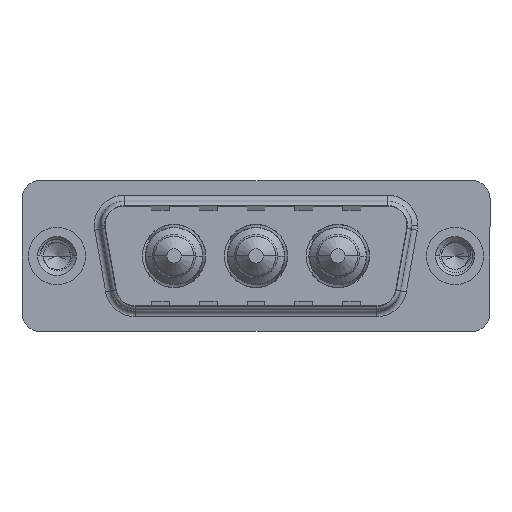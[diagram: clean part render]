
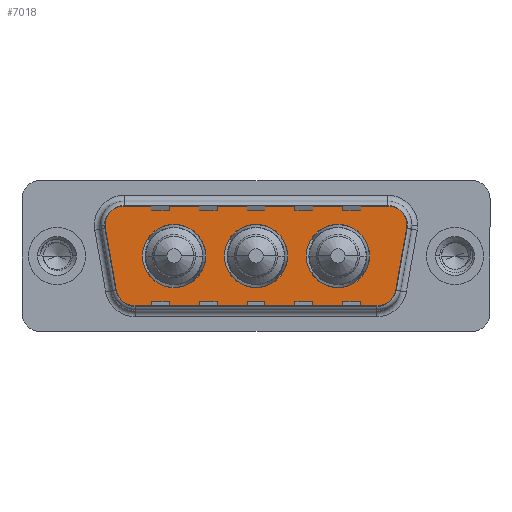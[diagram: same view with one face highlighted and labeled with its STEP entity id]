
A CAD part, top view. The second image highlights one B-rep face of the part: STEP entity #7018.
In plain terms, the highlighted planar face has unit normal (0, 0, 1).
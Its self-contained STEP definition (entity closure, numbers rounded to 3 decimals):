
#6 = ORIENTED_EDGE ( 'NONE', *, *, #17753, .F. ) ;
#255 = CARTESIAN_POINT ( 'NONE',  ( 27.889, 2.9, 0. ) ) ;
#508 = CARTESIAN_POINT ( 'NONE',  ( 26.866, -2.9, 0. ) ) ;
#738 = DIRECTION ( 'NONE',  ( 1., 0., 0. ) ) ;
#1207 = FACE_OUTER_BOUND ( 'NONE', #15820, .T. ) ;
#1309 = DIRECTION ( 'NONE',  ( 0., 0., 1. ) ) ;
#1319 = CARTESIAN_POINT ( 'NONE',  ( 3.441, 2.553, 0. ) ) ;
#1426 = CARTESIAN_POINT ( 'NONE',  ( 28.836, -3.247, 0. ) ) ;
#1541 = VERTEX_POINT ( 'NONE', #5702 ) ;
#1568 = ORIENTED_EDGE ( 'NONE', *, *, #14304, .F. ) ;
#1627 = DIRECTION ( 'NONE',  ( -1., 0., 0. ) ) ;
#1769 = AXIS2_PLACEMENT_3D ( 'NONE', #3737, #13421, #5131 ) ;
#1895 = DIRECTION ( 'NONE',  ( 1., 0., 0. ) ) ;
#1977 = DIRECTION ( 'NONE',  ( 0., 0., 1. ) ) ;
#2064 = FACE_BOUND ( 'NONE', #12384, .T. ) ;
#2114 = CARTESIAN_POINT ( 'NONE',  ( 26.15, 0., 0. ) ) ;
#2203 = CARTESIAN_POINT ( 'NONE',  ( 6.434, -4.9, 0. ) ) ;
#2227 = ORIENTED_EDGE ( 'NONE', *, *, #14555, .T. ) ;
#2280 = CIRCLE ( 'NONE', #8148, 2.65 ) ;
#2537 = CIRCLE ( 'NONE', #9273, 2. ) ;
#2560 = VECTOR ( 'NONE', #9613, 1000. ) ;
#2622 = DIRECTION ( 'NONE',  ( 0., 0., 1. ) ) ;
#2796 = CARTESIAN_POINT ( 'NONE',  ( 6.434, -2.9, 0. ) ) ;
#2986 = VERTEX_POINT ( 'NONE', #2114 ) ;
#3017 = AXIS2_PLACEMENT_3D ( 'NONE', #8143, #1309, #10999 ) ;
#3078 = CARTESIAN_POINT ( 'NONE',  ( 5.411, 4.9, 0. ) ) ;
#3218 = ORIENTED_EDGE ( 'NONE', *, *, #4430, .T. ) ;
#3278 = AXIS2_PLACEMENT_3D ( 'NONE', #10917, #2622, #12318 ) ;
#3507 = CIRCLE ( 'NONE', #1769, 2. ) ;
#3562 = CARTESIAN_POINT ( 'NONE',  ( 29.859, 2.553, 0. ) ) ;
#3585 = ORIENTED_EDGE ( 'NONE', *, *, #9529, .T. ) ;
#3737 = CARTESIAN_POINT ( 'NONE',  ( 27.889, 2.9, 0. ) ) ;
#3794 = CARTESIAN_POINT ( 'NONE',  ( 26.866, -4.9, 0. ) ) ;
#4086 = DIRECTION ( 'NONE',  ( 0., 0., 1. ) ) ;
#4202 = DIRECTION ( 'NONE',  ( -1., 0., 0. ) ) ;
#4228 = VERTEX_POINT ( 'NONE', #14445 ) ;
#4291 = CARTESIAN_POINT ( 'NONE',  ( 27.889, 4.9, 0. ) ) ;
#4430 = EDGE_CURVE ( 'NONE', #6478, #1541, #11515, .T. ) ;
#4602 = AXIS2_PLACEMENT_3D ( 'NONE', #10273, #1977, #11667 ) ;
#4649 = AXIS2_PLACEMENT_3D ( 'NONE', #12376, #4086, #13775 ) ;
#5131 = DIRECTION ( 'NONE',  ( -1., 0., 0. ) ) ;
#5272 = ORIENTED_EDGE ( 'NONE', *, *, #14531, .F. ) ;
#5702 = CARTESIAN_POINT ( 'NONE',  ( 3.441, 2.553, 0. ) ) ;
#5924 = CARTESIAN_POINT ( 'NONE',  ( 12.45, 0., 0. ) ) ;
#6120 = VERTEX_POINT ( 'NONE', #10909 ) ;
#6264 = ORIENTED_EDGE ( 'NONE', *, *, #10091, .F. ) ;
#6368 = DIRECTION ( 'NONE',  ( 0.174, 0.985, 0. ) ) ;
#6478 = VERTEX_POINT ( 'NONE', #3078 ) ;
#6599 = CARTESIAN_POINT ( 'NONE',  ( 5.411, 2.9, 0. ) ) ;
#6802 = CARTESIAN_POINT ( 'NONE',  ( 14., 0., 0. ) ) ;
#7018 = ADVANCED_FACE ( 'NONE', ( #11812, #8566, #2064, #1207 ), #16489, .T. ) ;
#7103 = CIRCLE ( 'NONE', #4649, 2.65 ) ;
#7145 = EDGE_LOOP ( 'NONE', ( #7557, #6264 ) ) ;
#7215 = VERTEX_POINT ( 'NONE', #1426 ) ;
#7420 = EDGE_CURVE ( 'NONE', #15834, #7215, #10281, .T. ) ;
#7491 = CARTESIAN_POINT ( 'NONE',  ( 23.5, 0., 0. ) ) ;
#7525 = AXIS2_PLACEMENT_3D ( 'NONE', #15916, #7639, #17315 ) ;
#7557 = ORIENTED_EDGE ( 'NONE', *, *, #12801, .F. ) ;
#7639 = DIRECTION ( 'NONE',  ( 0., 0., 1. ) ) ;
#7760 = LINE ( 'NONE', #14717, #14684 ) ;
#7969 = DIRECTION ( 'NONE',  ( 1., 0., 0. ) ) ;
#8143 = CARTESIAN_POINT ( 'NONE',  ( 26.866, -2.9, 0. ) ) ;
#8148 = AXIS2_PLACEMENT_3D ( 'NONE', #7491, #17171, #8862 ) ;
#8149 = ORIENTED_EDGE ( 'NONE', *, *, #17123, .T. ) ;
#8280 = AXIS2_PLACEMENT_3D ( 'NONE', #17295, #8998, #738 ) ;
#8478 = CIRCLE ( 'NONE', #3278, 2.65 ) ;
#8566 = FACE_BOUND ( 'NONE', #7145, .T. ) ;
#8862 = DIRECTION ( 'NONE',  ( 1., 0., 0. ) ) ;
#8873 = AXIS2_PLACEMENT_3D ( 'NONE', #6599, #16255, #7969 ) ;
#8998 = DIRECTION ( 'NONE',  ( 0., 0., 1. ) ) ;
#9211 = DIRECTION ( 'NONE',  ( -1., 0., 0. ) ) ;
#9273 = AXIS2_PLACEMENT_3D ( 'NONE', #2796, #12490, #4202 ) ;
#9278 = AXIS2_PLACEMENT_3D ( 'NONE', #255, #9926, #1627 ) ;
#9506 = CIRCLE ( 'NONE', #7525, 2.65 ) ;
#9520 = CARTESIAN_POINT ( 'NONE',  ( 6.434, -4.9, 0. ) ) ;
#9529 = EDGE_CURVE ( 'NONE', #12330, #16066, #3507, .T. ) ;
#9613 = DIRECTION ( 'NONE',  ( 0.174, -0.985, 0. ) ) ;
#9926 = DIRECTION ( 'NONE',  ( 0., 0., 1. ) ) ;
#9934 = LINE ( 'NONE', #1319, #2560 ) ;
#10091 = EDGE_CURVE ( 'NONE', #4228, #2986, #9506, .T. ) ;
#10186 = DIRECTION ( 'NONE',  ( 0., 0., 1. ) ) ;
#10207 = ORIENTED_EDGE ( 'NONE', *, *, #10208, .T. ) ;
#10208 = EDGE_CURVE ( 'NONE', #16066, #6478, #7760, .T. ) ;
#10273 = CARTESIAN_POINT ( 'NONE',  ( 16.65, 0., 0. ) ) ;
#10281 = CIRCLE ( 'NONE', #15645, 2. ) ;
#10834 = VERTEX_POINT ( 'NONE', #6802 ) ;
#10909 = CARTESIAN_POINT ( 'NONE',  ( 4.464, -3.247, 0. ) ) ;
#10917 = CARTESIAN_POINT ( 'NONE',  ( 9.8, 0., 0. ) ) ;
#10999 = DIRECTION ( 'NONE',  ( 1., 0., 0. ) ) ;
#11085 = EDGE_CURVE ( 'NONE', #11419, #12330, #14884, .T. ) ;
#11299 = CARTESIAN_POINT ( 'NONE',  ( 29.889, 2.9, 0. ) ) ;
#11419 = VERTEX_POINT ( 'NONE', #17453 ) ;
#11515 = CIRCLE ( 'NONE', #8873, 2. ) ;
#11558 = ORIENTED_EDGE ( 'NONE', *, *, #12901, .T. ) ;
#11641 = ORIENTED_EDGE ( 'NONE', *, *, #11085, .T. ) ;
#11667 = DIRECTION ( 'NONE',  ( 1., 0., 0. ) ) ;
#11812 = FACE_BOUND ( 'NONE', #16914, .T. ) ;
#12172 = ORIENTED_EDGE ( 'NONE', *, *, #7420, .T. ) ;
#12173 = LINE ( 'NONE', #9520, #14527 ) ;
#12258 = VERTEX_POINT ( 'NONE', #13910 ) ;
#12318 = DIRECTION ( 'NONE',  ( 1., 0., 0. ) ) ;
#12330 = VERTEX_POINT ( 'NONE', #11299 ) ;
#12365 = VERTEX_POINT ( 'NONE', #16898 ) ;
#12376 = CARTESIAN_POINT ( 'NONE',  ( 16.65, 0., 0. ) ) ;
#12384 = EDGE_LOOP ( 'NONE', ( #5272, #1568 ) ) ;
#12412 = VERTEX_POINT ( 'NONE', #5924 ) ;
#12490 = DIRECTION ( 'NONE',  ( 0., 0., 1. ) ) ;
#12552 = ORIENTED_EDGE ( 'NONE', *, *, #17822, .T. ) ;
#12801 = EDGE_CURVE ( 'NONE', #2986, #4228, #2280, .T. ) ;
#12901 = EDGE_CURVE ( 'NONE', #7215, #11419, #12902, .T. ) ;
#12902 = LINE ( 'NONE', #3562, #15678 ) ;
#13421 = DIRECTION ( 'NONE',  ( 0., 0., 1. ) ) ;
#13716 = DIRECTION ( 'NONE',  ( 1., 0., 0. ) ) ;
#13775 = DIRECTION ( 'NONE',  ( 1., 0., 0. ) ) ;
#13850 = CIRCLE ( 'NONE', #4602, 2.65 ) ;
#13910 = CARTESIAN_POINT ( 'NONE',  ( 19.3, 0., 0. ) ) ;
#13917 = CIRCLE ( 'NONE', #8280, 2.65 ) ;
#14304 = EDGE_CURVE ( 'NONE', #12365, #12412, #13917, .T. ) ;
#14445 = CARTESIAN_POINT ( 'NONE',  ( 20.85, 0., 0. ) ) ;
#14527 = VECTOR ( 'NONE', #13716, 1000. ) ;
#14531 = EDGE_CURVE ( 'NONE', #12412, #12365, #8478, .T. ) ;
#14555 = EDGE_CURVE ( 'NONE', #17257, #15834, #12173, .T. ) ;
#14565 = ORIENTED_EDGE ( 'NONE', *, *, #16737, .F. ) ;
#14684 = VECTOR ( 'NONE', #9211, 1000. ) ;
#14717 = CARTESIAN_POINT ( 'NONE',  ( 5.411, 4.9, 0. ) ) ;
#14884 = CIRCLE ( 'NONE', #9278, 2. ) ;
#15645 = AXIS2_PLACEMENT_3D ( 'NONE', #508, #10186, #1895 ) ;
#15678 = VECTOR ( 'NONE', #6368, 1000. ) ;
#15820 = EDGE_LOOP ( 'NONE', ( #12172, #11558, #11641, #3585, #10207, #3218, #8149, #12552, #2227 ) ) ;
#15834 = VERTEX_POINT ( 'NONE', #3794 ) ;
#15916 = CARTESIAN_POINT ( 'NONE',  ( 23.5, 0., 0. ) ) ;
#16066 = VERTEX_POINT ( 'NONE', #4291 ) ;
#16255 = DIRECTION ( 'NONE',  ( 0., 0., 1. ) ) ;
#16489 = PLANE ( 'NONE',  #3017 ) ;
#16737 = EDGE_CURVE ( 'NONE', #10834, #12258, #13850, .T. ) ;
#16898 = CARTESIAN_POINT ( 'NONE',  ( 7.15, 0., 0. ) ) ;
#16914 = EDGE_LOOP ( 'NONE', ( #6, #14565 ) ) ;
#17123 = EDGE_CURVE ( 'NONE', #1541, #6120, #9934, .T. ) ;
#17171 = DIRECTION ( 'NONE',  ( 0., 0., 1. ) ) ;
#17257 = VERTEX_POINT ( 'NONE', #2203 ) ;
#17295 = CARTESIAN_POINT ( 'NONE',  ( 9.8, 0., 0. ) ) ;
#17315 = DIRECTION ( 'NONE',  ( 1., 0., 0. ) ) ;
#17453 = CARTESIAN_POINT ( 'NONE',  ( 29.859, 2.553, 0. ) ) ;
#17753 = EDGE_CURVE ( 'NONE', #12258, #10834, #7103, .T. ) ;
#17822 = EDGE_CURVE ( 'NONE', #6120, #17257, #2537, .T. ) ;
